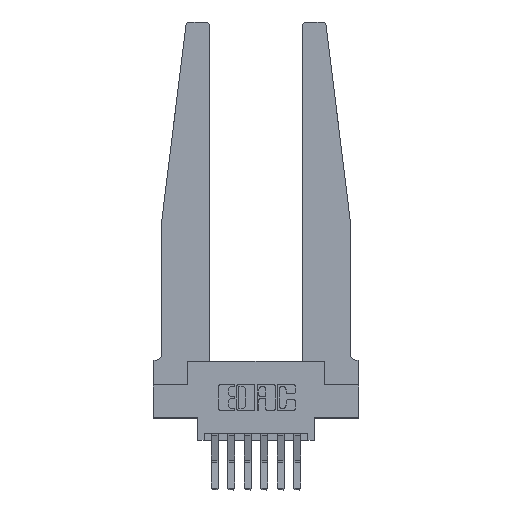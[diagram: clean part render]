
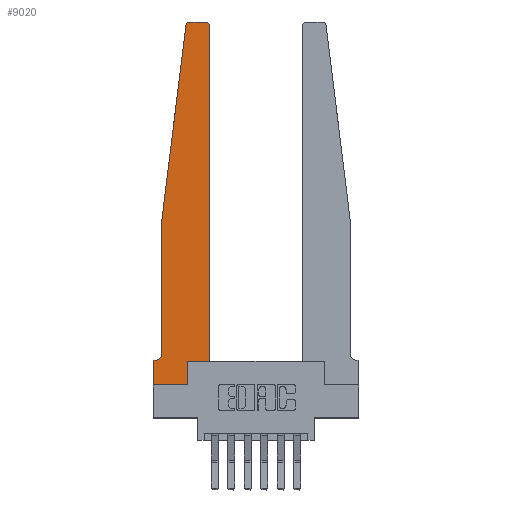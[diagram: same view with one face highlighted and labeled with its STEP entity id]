
A CAD part, top view. The second image highlights one B-rep face of the part: STEP entity #9020.
In plain terms, the highlighted planar face has unit normal (0, 0, 1).
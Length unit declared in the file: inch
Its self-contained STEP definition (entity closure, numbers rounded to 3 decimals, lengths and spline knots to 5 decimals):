
#31 = LINE ( 'NONE', #8944, #10442 ) ;
#113 = EDGE_CURVE ( 'NONE', #12673, #6771, #13505, .T. ) ;
#182 = VERTEX_POINT ( 'NONE', #13840 ) ;
#203 = LINE ( 'NONE', #6942, #11363 ) ;
#293 = DIRECTION ( 'NONE',  ( 0., 1., 0. ) ) ;
#405 = CARTESIAN_POINT ( 'NONE',  ( 0.395, 2.72, 0.37 ) ) ;
#731 = DIRECTION ( 'NONE',  ( 1., 0., 0. ) ) ;
#1011 = DIRECTION ( 'NONE',  ( 1., 0., 0. ) ) ;
#1046 = LINE ( 'NONE', #7440, #6543 ) ;
#1136 = CARTESIAN_POINT ( 'NONE',  ( 0.24675, 2.72367, 0.37 ) ) ;
#1180 = EDGE_CURVE ( 'NONE', #3515, #10850, #2013, .T. ) ;
#1561 = DIRECTION ( 'NONE',  ( 1., 0., 0. ) ) ;
#1571 = DIRECTION ( 'NONE',  ( 1., 0., 0. ) ) ;
#1674 = CARTESIAN_POINT ( 'NONE',  ( 0., 0., 0.37 ) ) ;
#1676 = CARTESIAN_POINT ( 'NONE',  ( 0.2605, 0., 0.37 ) ) ;
#1808 = ORIENTED_EDGE ( 'NONE', *, *, #12354, .T. ) ;
#2013 = CIRCLE ( 'NONE', #3168, 0.03 ) ;
#2376 = VERTEX_POINT ( 'NONE', #7309 ) ;
#2462 = CARTESIAN_POINT ( 'NONE',  ( 0., 0., 0.37 ) ) ;
#2695 = VECTOR ( 'NONE', #8044, 39.37008 ) ;
#2795 = DIRECTION ( 'NONE',  ( -1., 0., 0. ) ) ;
#3066 = CARTESIAN_POINT ( 'NONE',  ( 0.065, 1.25, 0.37 ) ) ;
#3168 = AXIS2_PLACEMENT_3D ( 'NONE', #7487, #5544, #1011 ) ;
#3385 = VECTOR ( 'NONE', #11893, 39.37008 ) ;
#3515 = VERTEX_POINT ( 'NONE', #9982 ) ;
#3692 = ORIENTED_EDGE ( 'NONE', *, *, #1180, .T. ) ;
#3827 = CARTESIAN_POINT ( 'NONE',  ( 0.425, 0.18, 0.37 ) ) ;
#3878 = EDGE_CURVE ( 'NONE', #10609, #2376, #11754, .T. ) ;
#4010 = LINE ( 'NONE', #12634, #4015 ) ;
#4015 = VECTOR ( 'NONE', #2795, 39.37008 ) ;
#4294 = EDGE_CURVE ( 'NONE', #6771, #8930, #6436, .T. ) ;
#4361 = DIRECTION ( 'NONE',  ( 0., -1., 0. ) ) ;
#4793 = ORIENTED_EDGE ( 'NONE', *, *, #10210, .T. ) ;
#4928 = AXIS2_PLACEMENT_3D ( 'NONE', #12006, #7780, #10861 ) ;
#5146 = DIRECTION ( 'NONE',  ( 0., 1., 0. ) ) ;
#5149 = CARTESIAN_POINT ( 'NONE',  ( 0.425, 0.18, 0.37 ) ) ;
#5278 = ORIENTED_EDGE ( 'NONE', *, *, #13821, .T. ) ;
#5544 = DIRECTION ( 'NONE',  ( 0., 0., 1. ) ) ;
#5859 = CARTESIAN_POINT ( 'NONE',  ( 0., 0.1875, 0.37 ) ) ;
#5867 = CIRCLE ( 'NONE', #12283, 0.03 ) ;
#6436 = LINE ( 'NONE', #7510, #3385 ) ;
#6543 = VECTOR ( 'NONE', #5146, 39.37008 ) ;
#6634 = EDGE_CURVE ( 'NONE', #10850, #10609, #31, .T. ) ;
#6771 = VERTEX_POINT ( 'NONE', #1674 ) ;
#6908 = CARTESIAN_POINT ( 'NONE',  ( 0.425, 2.72, 0.37 ) ) ;
#6942 = CARTESIAN_POINT ( 'NONE',  ( 0.425, 0.18, 0.37 ) ) ;
#7309 = CARTESIAN_POINT ( 'NONE',  ( 0.065, 0.2375, 0.37 ) ) ;
#7310 = CARTESIAN_POINT ( 'NONE',  ( 0.015, 0.1875, 0.37 ) ) ;
#7440 = CARTESIAN_POINT ( 'NONE',  ( 0.2605, 0.18, 0.37 ) ) ;
#7487 = CARTESIAN_POINT ( 'NONE',  ( 0.27653, 2.72, 0.37 ) ) ;
#7510 = CARTESIAN_POINT ( 'NONE',  ( 0., 0., 0.37 ) ) ;
#7618 = ORIENTED_EDGE ( 'NONE', *, *, #13740, .T. ) ;
#7780 = DIRECTION ( 'NONE',  ( 0., 0., -1. ) ) ;
#8044 = DIRECTION ( 'NONE',  ( 0., -1., 0. ) ) ;
#8061 = VERTEX_POINT ( 'NONE', #12945 ) ;
#8281 = ORIENTED_EDGE ( 'NONE', *, *, #10131, .T. ) ;
#8567 = CARTESIAN_POINT ( 'NONE',  ( 0., 0.1875, 0.37 ) ) ;
#8665 = AXIS2_PLACEMENT_3D ( 'NONE', #8567, #14016, #731 ) ;
#8930 = VERTEX_POINT ( 'NONE', #1676 ) ;
#8944 = CARTESIAN_POINT ( 'NONE',  ( 0.065, 1.25, 0.37 ) ) ;
#9020 = ADVANCED_FACE ( 'NONE', ( #9797 ), #12946, .T. ) ;
#9192 = ORIENTED_EDGE ( 'NONE', *, *, #4294, .T. ) ;
#9553 = ORIENTED_EDGE ( 'NONE', *, *, #6634, .T. ) ;
#9656 = EDGE_CURVE ( 'NONE', #13567, #12673, #4010, .T. ) ;
#9797 = FACE_OUTER_BOUND ( 'NONE', #14013, .T. ) ;
#9812 = VECTOR ( 'NONE', #4361, 39.37008 ) ;
#9982 = CARTESIAN_POINT ( 'NONE',  ( 0.27653, 2.75, 0.37 ) ) ;
#10072 = ORIENTED_EDGE ( 'NONE', *, *, #3878, .T. ) ;
#10131 = EDGE_CURVE ( 'NONE', #2376, #13567, #11132, .T. ) ;
#10205 = VECTOR ( 'NONE', #293, 39.37008 ) ;
#10210 = EDGE_CURVE ( 'NONE', #12456, #10215, #13580, .T. ) ;
#10215 = VERTEX_POINT ( 'NONE', #6908 ) ;
#10318 = DIRECTION ( 'NONE',  ( 0., 0., 1. ) ) ;
#10361 = ORIENTED_EDGE ( 'NONE', *, *, #9656, .T. ) ;
#10442 = VECTOR ( 'NONE', #12171, 39.37008 ) ;
#10609 = VERTEX_POINT ( 'NONE', #12363 ) ;
#10850 = VERTEX_POINT ( 'NONE', #1136 ) ;
#10861 = DIRECTION ( 'NONE',  ( -1., 0., 0. ) ) ;
#10953 = ORIENTED_EDGE ( 'NONE', *, *, #12659, .T. ) ;
#11037 = CARTESIAN_POINT ( 'NONE',  ( 0.25, 2.75, 0.37 ) ) ;
#11132 = CIRCLE ( 'NONE', #4928, 0.05 ) ;
#11363 = VECTOR ( 'NONE', #1571, 39.37008 ) ;
#11428 = ORIENTED_EDGE ( 'NONE', *, *, #113, .T. ) ;
#11582 = VECTOR ( 'NONE', #13261, 39.37008 ) ;
#11754 = LINE ( 'NONE', #3066, #9812 ) ;
#11893 = DIRECTION ( 'NONE',  ( 1., 0., 0. ) ) ;
#12006 = CARTESIAN_POINT ( 'NONE',  ( 0.015, 0.2375, 0.37 ) ) ;
#12025 = LINE ( 'NONE', #11037, #11582 ) ;
#12171 = DIRECTION ( 'NONE',  ( -0.122, -0.992, 0. ) ) ;
#12283 = AXIS2_PLACEMENT_3D ( 'NONE', #405, #10318, #1561 ) ;
#12354 = EDGE_CURVE ( 'NONE', #8061, #12456, #203, .T. ) ;
#12363 = CARTESIAN_POINT ( 'NONE',  ( 0.065, 1.25, 0.37 ) ) ;
#12456 = VERTEX_POINT ( 'NONE', #5149 ) ;
#12634 = CARTESIAN_POINT ( 'NONE',  ( 0.065, 0.1875, 0.37 ) ) ;
#12659 = EDGE_CURVE ( 'NONE', #10215, #182, #5867, .T. ) ;
#12673 = VERTEX_POINT ( 'NONE', #5859 ) ;
#12945 = CARTESIAN_POINT ( 'NONE',  ( 0.2605, 0.18, 0.37 ) ) ;
#12946 = PLANE ( 'NONE',  #8665 ) ;
#13261 = DIRECTION ( 'NONE',  ( -1., 0., 0. ) ) ;
#13505 = LINE ( 'NONE', #2462, #2695 ) ;
#13567 = VERTEX_POINT ( 'NONE', #7310 ) ;
#13580 = LINE ( 'NONE', #3827, #10205 ) ;
#13740 = EDGE_CURVE ( 'NONE', #8930, #8061, #1046, .T. ) ;
#13821 = EDGE_CURVE ( 'NONE', #182, #3515, #12025, .T. ) ;
#13840 = CARTESIAN_POINT ( 'NONE',  ( 0.395, 2.75, 0.37 ) ) ;
#14013 = EDGE_LOOP ( 'NONE', ( #5278, #3692, #9553, #10072, #8281, #10361, #11428, #9192, #7618, #1808, #4793, #10953 ) ) ;
#14016 = DIRECTION ( 'NONE',  ( 0., 0., 1. ) ) ;
